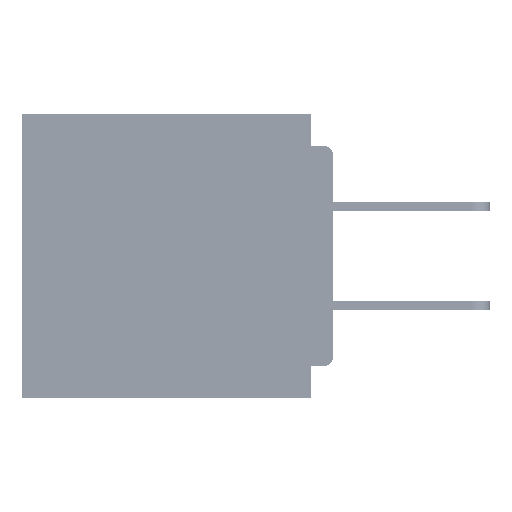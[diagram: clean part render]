
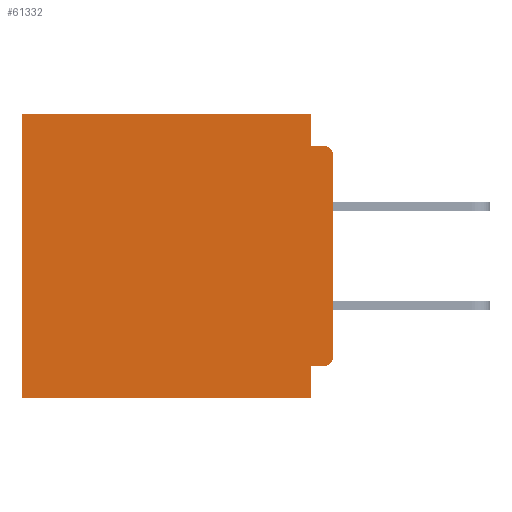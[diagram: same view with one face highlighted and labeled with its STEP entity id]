
A CAD part, left-side view. The second image highlights one B-rep face of the part: STEP entity #61332.
In plain terms, the highlighted planar face has unit normal (-1, 0, 0).
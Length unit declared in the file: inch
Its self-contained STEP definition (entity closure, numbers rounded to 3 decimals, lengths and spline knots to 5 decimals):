
#538 = PLANE ( 'NONE',  #46106 ) ;
#883 = VECTOR ( 'NONE', #61123, 39.37008 ) ;
#889 = ORIENTED_EDGE ( 'NONE', *, *, #56908, .T. ) ;
#902 = VERTEX_POINT ( 'NONE', #52975 ) ;
#964 = EDGE_CURVE ( 'NONE', #38425, #59249, #61879, .T. ) ;
#1501 = VERTEX_POINT ( 'NONE', #57025 ) ;
#1598 = DIRECTION ( 'NONE',  ( -1., 0., 0. ) ) ;
#1676 = CARTESIAN_POINT ( 'NONE',  ( 0.3, 0.031, -0.4 ) ) ;
#2384 = CARTESIAN_POINT ( 'NONE',  ( 0.3, 0., -0.045 ) ) ;
#4161 = ORIENTED_EDGE ( 'NONE', *, *, #29364, .F. ) ;
#5976 = DIRECTION ( 'NONE',  ( 0., 1., 0. ) ) ;
#6362 = CARTESIAN_POINT ( 'NONE',  ( 0.3, 0., -0.4 ) ) ;
#8148 = EDGE_CURVE ( 'NONE', #57006, #1501, #53721, .T. ) ;
#8578 = EDGE_CURVE ( 'NONE', #57006, #20251, #42463, .T. ) ;
#9193 = VERTEX_POINT ( 'NONE', #1676 ) ;
#9731 = CARTESIAN_POINT ( 'NONE',  ( 0.3, 0.031, -0.4 ) ) ;
#10264 = DIRECTION ( 'NONE',  ( 0., 0., -1. ) ) ;
#10601 = VECTOR ( 'NONE', #19497, 39.37008 ) ;
#10843 = AXIS2_PLACEMENT_3D ( 'NONE', #26747, #52343, #30461 ) ;
#12100 = ORIENTED_EDGE ( 'NONE', *, *, #8578, .T. ) ;
#12672 = ORIENTED_EDGE ( 'NONE', *, *, #30227, .F. ) ;
#14323 = VECTOR ( 'NONE', #55656, 39.37008 ) ;
#15435 = LINE ( 'NONE', #34972, #26839 ) ;
#15565 = CIRCLE ( 'NONE', #37489, 0.015 ) ;
#15835 = VECTOR ( 'NONE', #25875, 39.37008 ) ;
#16211 = FACE_OUTER_BOUND ( 'NONE', #18548, .T. ) ;
#16483 = CARTESIAN_POINT ( 'NONE',  ( 0.3, 0., -0.34 ) ) ;
#16809 = VECTOR ( 'NONE', #60299, 39.37008 ) ;
#18324 = LINE ( 'NONE', #32461, #883 ) ;
#18548 = EDGE_LOOP ( 'NONE', ( #4161, #30529, #29803, #62382, #12100, #889, #23896, #12672, #27498, #40715 ) ) ;
#18673 = VERTEX_POINT ( 'NONE', #41727 ) ;
#19497 = DIRECTION ( 'NONE',  ( 0., 0., -1. ) ) ;
#20251 = VERTEX_POINT ( 'NONE', #48354 ) ;
#23896 = ORIENTED_EDGE ( 'NONE', *, *, #45732, .F. ) ;
#24008 = VERTEX_POINT ( 'NONE', #25538 ) ;
#25538 = CARTESIAN_POINT ( 'NONE',  ( 0.3, 0.437, -0.4 ) ) ;
#25541 = DIRECTION ( 'NONE',  ( 0., 1., 0. ) ) ;
#25875 = DIRECTION ( 'NONE',  ( 0., 1., 0. ) ) ;
#26747 = CARTESIAN_POINT ( 'NONE',  ( 0.3, 0.015, -0.34 ) ) ;
#26839 = VECTOR ( 'NONE', #25541, 39.37008 ) ;
#26954 = CARTESIAN_POINT ( 'NONE',  ( 0.3, 0.437, -0.4 ) ) ;
#27229 = LINE ( 'NONE', #26954, #14323 ) ;
#27498 = ORIENTED_EDGE ( 'NONE', *, *, #36262, .F. ) ;
#28783 = LINE ( 'NONE', #6362, #15835 ) ;
#29364 = EDGE_CURVE ( 'NONE', #18673, #59249, #18324, .T. ) ;
#29694 = VECTOR ( 'NONE', #5976, 39.37008 ) ;
#29803 = ORIENTED_EDGE ( 'NONE', *, *, #36425, .F. ) ;
#30227 = EDGE_CURVE ( 'NONE', #38815, #9193, #37813, .T. ) ;
#30461 = DIRECTION ( 'NONE',  ( 0., 0., -1. ) ) ;
#30529 = ORIENTED_EDGE ( 'NONE', *, *, #41453, .T. ) ;
#30605 = VECTOR ( 'NONE', #36220, 39.37008 ) ;
#30643 = CARTESIAN_POINT ( 'NONE',  ( 0.3, 0.015, -0.06 ) ) ;
#32461 = CARTESIAN_POINT ( 'NONE',  ( 0.3, 0., -0.4 ) ) ;
#34226 = CARTESIAN_POINT ( 'NONE',  ( 0.3, 0.031, -0.355 ) ) ;
#34918 = CARTESIAN_POINT ( 'NONE',  ( 0.3, 0., 0. ) ) ;
#34972 = CARTESIAN_POINT ( 'NONE',  ( 0.3, 0., -0.355 ) ) ;
#35407 = DIRECTION ( 'NONE',  ( 0., 0., -1. ) ) ;
#35942 = CARTESIAN_POINT ( 'NONE',  ( 0.3, 0.015, -0.355 ) ) ;
#36220 = DIRECTION ( 'NONE',  ( 0., -1., 0. ) ) ;
#36262 = EDGE_CURVE ( 'NONE', #38425, #38815, #15435, .T. ) ;
#36425 = EDGE_CURVE ( 'NONE', #1501, #902, #44840, .T. ) ;
#37489 = AXIS2_PLACEMENT_3D ( 'NONE', #30643, #1598, #35407 ) ;
#37813 = LINE ( 'NONE', #9731, #10601 ) ;
#38425 = VERTEX_POINT ( 'NONE', #35942 ) ;
#38815 = VERTEX_POINT ( 'NONE', #34226 ) ;
#39000 = DIRECTION ( 'NONE',  ( 1., 0., 0. ) ) ;
#40715 = ORIENTED_EDGE ( 'NONE', *, *, #964, .T. ) ;
#41453 = EDGE_CURVE ( 'NONE', #18673, #902, #15565, .T. ) ;
#41727 = CARTESIAN_POINT ( 'NONE',  ( 0.3, 0., -0.06 ) ) ;
#42084 = CARTESIAN_POINT ( 'NONE',  ( 0.3, 0.031, 0. ) ) ;
#42463 = LINE ( 'NONE', #34918, #29694 ) ;
#44840 = LINE ( 'NONE', #2384, #30605 ) ;
#45732 = EDGE_CURVE ( 'NONE', #9193, #24008, #28783, .T. ) ;
#46106 = AXIS2_PLACEMENT_3D ( 'NONE', #48615, #39000, #10264 ) ;
#48354 = CARTESIAN_POINT ( 'NONE',  ( 0.3, 0.437, 0. ) ) ;
#48615 = CARTESIAN_POINT ( 'NONE',  ( 0.3, 0., -0.4 ) ) ;
#50936 = CARTESIAN_POINT ( 'NONE',  ( 0.3, 0.031, 0. ) ) ;
#52343 = DIRECTION ( 'NONE',  ( -1., 0., 0. ) ) ;
#52975 = CARTESIAN_POINT ( 'NONE',  ( 0.3, 0.015, -0.045 ) ) ;
#53721 = LINE ( 'NONE', #50936, #16809 ) ;
#55656 = DIRECTION ( 'NONE',  ( 0., 0., -1. ) ) ;
#56908 = EDGE_CURVE ( 'NONE', #20251, #24008, #27229, .T. ) ;
#57006 = VERTEX_POINT ( 'NONE', #42084 ) ;
#57025 = CARTESIAN_POINT ( 'NONE',  ( 0.3, 0.031, -0.045 ) ) ;
#59249 = VERTEX_POINT ( 'NONE', #16483 ) ;
#60299 = DIRECTION ( 'NONE',  ( 0., 0., -1. ) ) ;
#61123 = DIRECTION ( 'NONE',  ( 0., 0., -1. ) ) ;
#61332 = ADVANCED_FACE ( 'NONE', ( #16211 ), #538, .F. ) ;
#61879 = CIRCLE ( 'NONE', #10843, 0.015 ) ;
#62382 = ORIENTED_EDGE ( 'NONE', *, *, #8148, .F. ) ;
